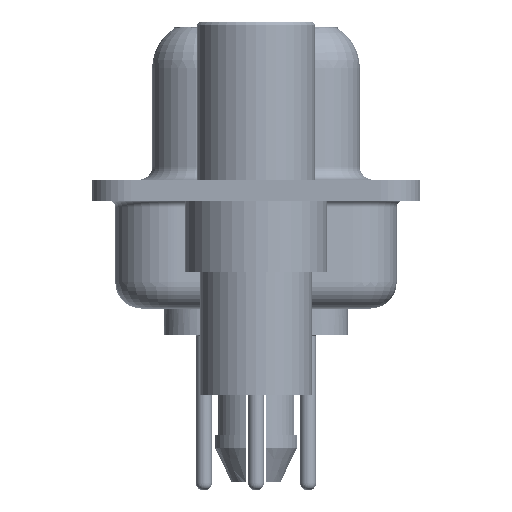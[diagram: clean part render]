
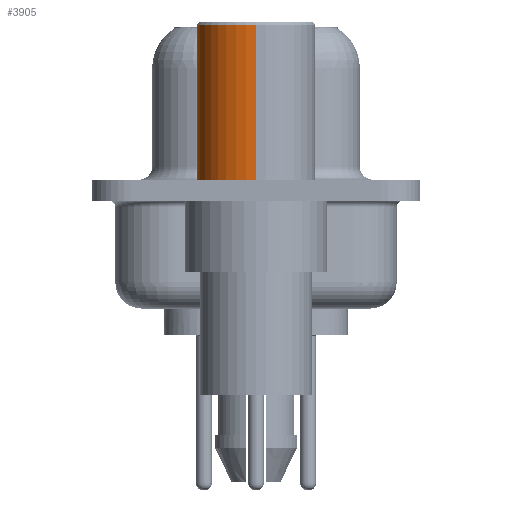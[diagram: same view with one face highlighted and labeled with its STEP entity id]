
A CAD part, left-side view. The second image highlights one B-rep face of the part: STEP entity #3905.
In plain terms, the highlighted cylindrical face has radius 2.25 mm (diameter 4.5 mm), a partial arc.
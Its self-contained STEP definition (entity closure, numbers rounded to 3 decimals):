
#101 = CARTESIAN_POINT ( 'NONE',  ( -2.25, 0., 0.4 ) ) ;
#328 = DIRECTION ( 'NONE',  ( 0., 0., 1. ) ) ;
#1074 = AXIS2_PLACEMENT_3D ( 'NONE', #25976, #37851, #11066 ) ;
#1734 = LINE ( 'NONE', #13702, #15848 ) ;
#2204 = VERTEX_POINT ( 'NONE', #101 ) ;
#2558 = AXIS2_PLACEMENT_3D ( 'NONE', #17899, #29821, #28060 ) ;
#3905 = ADVANCED_FACE ( 'NONE', ( #17712 ), #5937, .T. ) ;
#5127 = VECTOR ( 'NONE', #26782, 1000. ) ;
#5937 = CYLINDRICAL_SURFACE ( 'NONE', #2558, 2.25 ) ;
#6981 = EDGE_CURVE ( 'NONE', #16719, #13229, #13627, .T. ) ;
#7190 = ORIENTED_EDGE ( 'NONE', *, *, #29977, .F. ) ;
#7556 = VERTEX_POINT ( 'NONE', #35447 ) ;
#8360 = CARTESIAN_POINT ( 'NONE',  ( 0., 0., 0.4 ) ) ;
#8745 = DIRECTION ( 'NONE',  ( 1., 0., 0. ) ) ;
#8935 = DIRECTION ( 'NONE',  ( 0., 0., 1. ) ) ;
#9191 = ORIENTED_EDGE ( 'NONE', *, *, #28713, .T. ) ;
#9716 = CARTESIAN_POINT ( 'NONE',  ( 2.25, 0., 6.3 ) ) ;
#10958 = CARTESIAN_POINT ( 'NONE',  ( -2.25, 0., 6.3 ) ) ;
#11066 = DIRECTION ( 'NONE',  ( 1., 0., 0. ) ) ;
#13229 = VERTEX_POINT ( 'NONE', #10958 ) ;
#13627 = CIRCLE ( 'NONE', #1074, 2.25 ) ;
#13702 = CARTESIAN_POINT ( 'NONE',  ( 2.25, 0., 0.581 ) ) ;
#13879 = EDGE_CURVE ( 'NONE', #7556, #2204, #24710, .T. ) ;
#14839 = CARTESIAN_POINT ( 'NONE',  ( -2.25, 0., 0.581 ) ) ;
#15036 = ORIENTED_EDGE ( 'NONE', *, *, #13879, .T. ) ;
#15848 = VECTOR ( 'NONE', #328, 1000. ) ;
#16719 = VERTEX_POINT ( 'NONE', #9716 ) ;
#17712 = FACE_OUTER_BOUND ( 'NONE', #25204, .T. ) ;
#17899 = CARTESIAN_POINT ( 'NONE',  ( 0., 0., 0.581 ) ) ;
#24710 = CIRCLE ( 'NONE', #34678, 2.25 ) ;
#25204 = EDGE_LOOP ( 'NONE', ( #15036, #9191, #30210, #7190 ) ) ;
#25976 = CARTESIAN_POINT ( 'NONE',  ( 0., 0., 6.3 ) ) ;
#26782 = DIRECTION ( 'NONE',  ( 0., 0., 1. ) ) ;
#27694 = LINE ( 'NONE', #14839, #5127 ) ;
#28060 = DIRECTION ( 'NONE',  ( 1., 0., 0. ) ) ;
#28713 = EDGE_CURVE ( 'NONE', #2204, #13229, #27694, .T. ) ;
#29821 = DIRECTION ( 'NONE',  ( 0., 0., 1. ) ) ;
#29977 = EDGE_CURVE ( 'NONE', #7556, #16719, #1734, .T. ) ;
#30210 = ORIENTED_EDGE ( 'NONE', *, *, #6981, .F. ) ;
#34678 = AXIS2_PLACEMENT_3D ( 'NONE', #8360, #8935, #8745 ) ;
#35447 = CARTESIAN_POINT ( 'NONE',  ( 2.25, 0., 0.4 ) ) ;
#37851 = DIRECTION ( 'NONE',  ( 0., 0., 1. ) ) ;
